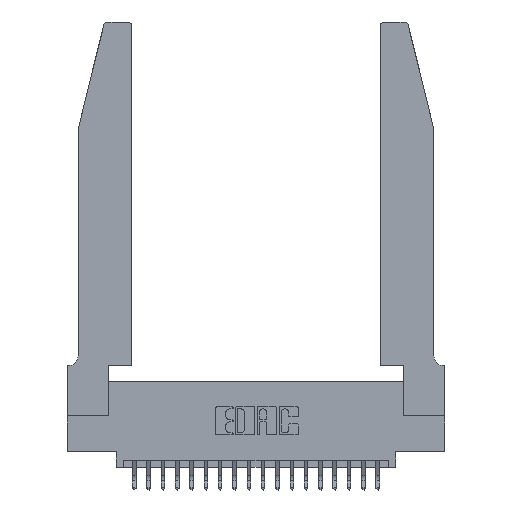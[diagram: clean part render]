
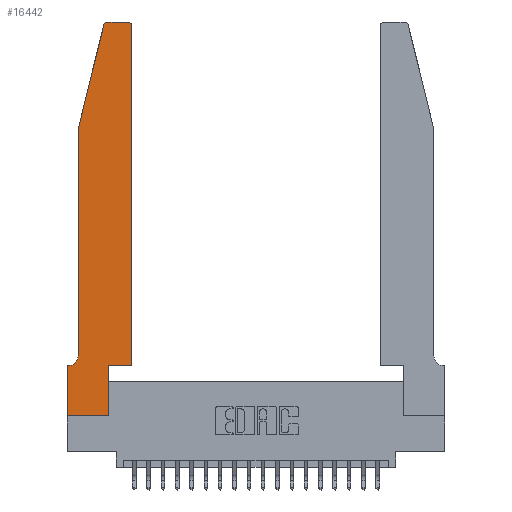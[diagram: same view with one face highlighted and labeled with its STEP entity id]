
A CAD part, top view. The second image highlights one B-rep face of the part: STEP entity #16442.
In plain terms, the highlighted planar face has unit normal (0, 0, 1).
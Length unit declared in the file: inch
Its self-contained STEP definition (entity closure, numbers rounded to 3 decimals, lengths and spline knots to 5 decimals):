
#451 = EDGE_CURVE ( 'NONE', #1033, #6479, #8527, .T. ) ;
#472 = AXIS2_PLACEMENT_3D ( 'NONE', #10761, #12486, #17719 ) ;
#688 = DIRECTION ( 'NONE',  ( -1., 0., 0. ) ) ;
#1016 = CARTESIAN_POINT ( 'NONE',  ( 0.4505, 0.35, 0.37 ) ) ;
#1033 = VERTEX_POINT ( 'NONE', #3049 ) ;
#1214 = CARTESIAN_POINT ( 'NONE',  ( 0.4505, 2.72, 0.37 ) ) ;
#1364 = CIRCLE ( 'NONE', #17484, 0.03 ) ;
#1631 = DIRECTION ( 'NONE',  ( 0., 0., 1. ) ) ;
#1675 = VECTOR ( 'NONE', #13191, 39.37008 ) ;
#2179 = ORIENTED_EDGE ( 'NONE', *, *, #10571, .T. ) ;
#2330 = CARTESIAN_POINT ( 'NONE',  ( 0.0755, 2., 0.37 ) ) ;
#2743 = ORIENTED_EDGE ( 'NONE', *, *, #21812, .T. ) ;
#2859 = ORIENTED_EDGE ( 'NONE', *, *, #17551, .T. ) ;
#3019 = CARTESIAN_POINT ( 'NONE',  ( 0.284, 2.75, 0.37 ) ) ;
#3049 = CARTESIAN_POINT ( 'NONE',  ( 0.4505, 0.35, 0.37 ) ) ;
#3287 = LINE ( 'NONE', #7608, #8148 ) ;
#3476 = VERTEX_POINT ( 'NONE', #19566 ) ;
#3482 = VECTOR ( 'NONE', #8973, 39.37008 ) ;
#4374 = VECTOR ( 'NONE', #4844, 39.37008 ) ;
#4474 = AXIS2_PLACEMENT_3D ( 'NONE', #19518, #21129, #17582 ) ;
#4844 = DIRECTION ( 'NONE',  ( 1., 0., 0. ) ) ;
#5006 = LINE ( 'NONE', #8746, #12027 ) ;
#5070 = CARTESIAN_POINT ( 'NONE',  ( 0.284, 2.72, 0.37 ) ) ;
#5339 = VERTEX_POINT ( 'NONE', #16541 ) ;
#5535 = VERTEX_POINT ( 'NONE', #18319 ) ;
#5745 = ORIENTED_EDGE ( 'NONE', *, *, #451, .T. ) ;
#6479 = VERTEX_POINT ( 'NONE', #1214 ) ;
#6680 = LINE ( 'NONE', #15370, #20506 ) ;
#7047 = VERTEX_POINT ( 'NONE', #3019 ) ;
#7049 = EDGE_CURVE ( 'NONE', #21660, #3476, #10654, .T. ) ;
#7441 = VECTOR ( 'NONE', #13601, 39.37008 ) ;
#7564 = CARTESIAN_POINT ( 'NONE',  ( 0.0755, 0.42, 0.37 ) ) ;
#7608 = CARTESIAN_POINT ( 'NONE',  ( 0.0755, 0.35, 0.37 ) ) ;
#7755 = DIRECTION ( 'NONE',  ( 0., 0., 1. ) ) ;
#7915 = ORIENTED_EDGE ( 'NONE', *, *, #21542, .T. ) ;
#8148 = VECTOR ( 'NONE', #688, 39.37008 ) ;
#8296 = CARTESIAN_POINT ( 'NONE',  ( 0.4505, 0.35, 0.37 ) ) ;
#8527 = LINE ( 'NONE', #8296, #7441 ) ;
#8729 = VERTEX_POINT ( 'NONE', #15754 ) ;
#8746 = CARTESIAN_POINT ( 'NONE',  ( 0.0755, 2., 0.37 ) ) ;
#8876 = LINE ( 'NONE', #2330, #3482 ) ;
#8973 = DIRECTION ( 'NONE',  ( -0.239, -0.971, 0. ) ) ;
#9193 = DIRECTION ( 'NONE',  ( 1., 0., 0. ) ) ;
#9433 = CARTESIAN_POINT ( 'NONE',  ( 0.4205, 2.72, 0.37 ) ) ;
#9958 = CIRCLE ( 'NONE', #4474, 0.07 ) ;
#10343 = DIRECTION ( 'NONE',  ( 0., -1., 0. ) ) ;
#10571 = EDGE_CURVE ( 'NONE', #3476, #13140, #6680, .T. ) ;
#10654 = LINE ( 'NONE', #11578, #19305 ) ;
#10761 = CARTESIAN_POINT ( 'NONE',  ( 0., 0.35, 0.37 ) ) ;
#10883 = ORIENTED_EDGE ( 'NONE', *, *, #12608, .T. ) ;
#10927 = LINE ( 'NONE', #15487, #21469 ) ;
#10935 = ORIENTED_EDGE ( 'NONE', *, *, #20262, .T. ) ;
#11008 = EDGE_CURVE ( 'NONE', #13140, #1033, #22265, .T. ) ;
#11578 = CARTESIAN_POINT ( 'NONE',  ( 0., 0., 0.37 ) ) ;
#11612 = ORIENTED_EDGE ( 'NONE', *, *, #17697, .T. ) ;
#11939 = DIRECTION ( 'NONE',  ( 0., -1., 0. ) ) ;
#12026 = VERTEX_POINT ( 'NONE', #17809 ) ;
#12027 = VECTOR ( 'NONE', #11939, 39.37008 ) ;
#12043 = ORIENTED_EDGE ( 'NONE', *, *, #11008, .T. ) ;
#12307 = AXIS2_PLACEMENT_3D ( 'NONE', #5070, #1631, #13895 ) ;
#12486 = DIRECTION ( 'NONE',  ( 0., 0., 1. ) ) ;
#12608 = EDGE_CURVE ( 'NONE', #16675, #5339, #8876, .T. ) ;
#13140 = VERTEX_POINT ( 'NONE', #14028 ) ;
#13191 = DIRECTION ( 'NONE',  ( -1., 0., 0. ) ) ;
#13601 = DIRECTION ( 'NONE',  ( 0., 1., 0. ) ) ;
#13895 = DIRECTION ( 'NONE',  ( 1., 0., 0. ) ) ;
#13898 = VERTEX_POINT ( 'NONE', #7564 ) ;
#14028 = CARTESIAN_POINT ( 'NONE',  ( 0.2865, 0.35, 0.37 ) ) ;
#14326 = CARTESIAN_POINT ( 'NONE',  ( 0., 0., 0.37 ) ) ;
#14426 = FACE_OUTER_BOUND ( 'NONE', #14594, .T. ) ;
#14594 = EDGE_LOOP ( 'NONE', ( #2743, #20995, #10883, #10935, #19770, #11612, #7915, #21939, #2179, #12043, #5745, #2859 ) ) ;
#15152 = DIRECTION ( 'NONE',  ( 0., 1., 0. ) ) ;
#15370 = CARTESIAN_POINT ( 'NONE',  ( 0.2865, 0.35, 0.37 ) ) ;
#15487 = CARTESIAN_POINT ( 'NONE',  ( 0., 0., 0.37 ) ) ;
#15754 = CARTESIAN_POINT ( 'NONE',  ( 0., 0.35, 0.37 ) ) ;
#16208 = PLANE ( 'NONE',  #472 ) ;
#16318 = LINE ( 'NONE', #18353, #1675 ) ;
#16442 = ADVANCED_FACE ( 'NONE', ( #14426 ), #16208, .T. ) ;
#16541 = CARTESIAN_POINT ( 'NONE',  ( 0.0755, 2., 0.37 ) ) ;
#16675 = VERTEX_POINT ( 'NONE', #20442 ) ;
#17484 = AXIS2_PLACEMENT_3D ( 'NONE', #9433, #7755, #9193 ) ;
#17551 = EDGE_CURVE ( 'NONE', #6479, #5535, #1364, .T. ) ;
#17582 = DIRECTION ( 'NONE',  ( -1., 0., 0. ) ) ;
#17697 = EDGE_CURVE ( 'NONE', #12026, #8729, #3287, .T. ) ;
#17715 = CIRCLE ( 'NONE', #12307, 0.03 ) ;
#17719 = DIRECTION ( 'NONE',  ( 1., 0., 0. ) ) ;
#17809 = CARTESIAN_POINT ( 'NONE',  ( 0.0055, 0.35, 0.37 ) ) ;
#18149 = EDGE_CURVE ( 'NONE', #13898, #12026, #9958, .T. ) ;
#18319 = CARTESIAN_POINT ( 'NONE',  ( 0.4205, 2.75, 0.37 ) ) ;
#18353 = CARTESIAN_POINT ( 'NONE',  ( 0.2605, 2.75, 0.37 ) ) ;
#19305 = VECTOR ( 'NONE', #20137, 39.37008 ) ;
#19518 = CARTESIAN_POINT ( 'NONE',  ( 0.0055, 0.42, 0.37 ) ) ;
#19566 = CARTESIAN_POINT ( 'NONE',  ( 0.2865, 0., 0.37 ) ) ;
#19770 = ORIENTED_EDGE ( 'NONE', *, *, #18149, .T. ) ;
#20137 = DIRECTION ( 'NONE',  ( 1., 0., 0. ) ) ;
#20262 = EDGE_CURVE ( 'NONE', #5339, #13898, #5006, .T. ) ;
#20267 = EDGE_CURVE ( 'NONE', #7047, #16675, #17715, .T. ) ;
#20442 = CARTESIAN_POINT ( 'NONE',  ( 0.25487, 2.72718, 0.37 ) ) ;
#20506 = VECTOR ( 'NONE', #15152, 39.37008 ) ;
#20995 = ORIENTED_EDGE ( 'NONE', *, *, #20267, .T. ) ;
#21129 = DIRECTION ( 'NONE',  ( 0., 0., -1. ) ) ;
#21469 = VECTOR ( 'NONE', #10343, 39.37008 ) ;
#21542 = EDGE_CURVE ( 'NONE', #8729, #21660, #10927, .T. ) ;
#21660 = VERTEX_POINT ( 'NONE', #14326 ) ;
#21812 = EDGE_CURVE ( 'NONE', #5535, #7047, #16318, .T. ) ;
#21939 = ORIENTED_EDGE ( 'NONE', *, *, #7049, .T. ) ;
#22265 = LINE ( 'NONE', #1016, #4374 ) ;
